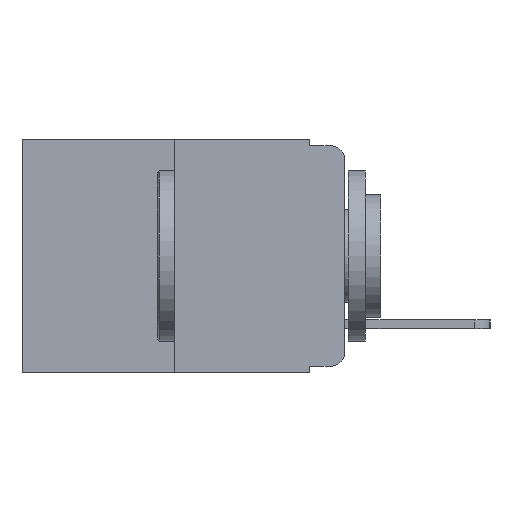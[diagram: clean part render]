
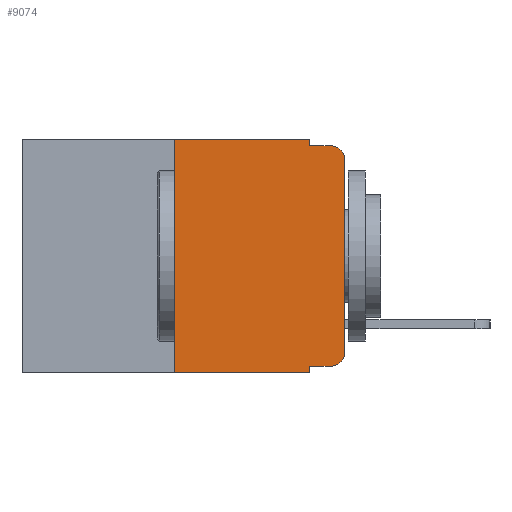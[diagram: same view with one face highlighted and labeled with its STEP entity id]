
A CAD part, left-side view. The second image highlights one B-rep face of the part: STEP entity #9074.
In plain terms, the highlighted planar face has unit normal (-1, 0, 0).
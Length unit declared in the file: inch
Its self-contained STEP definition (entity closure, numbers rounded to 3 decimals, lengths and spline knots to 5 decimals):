
#19 = EDGE_CURVE ( 'NONE', #1099, #6830, #603, .T. ) ;
#603 = LINE ( 'NONE', #7827, #10453 ) ;
#739 = CARTESIAN_POINT ( 'NONE',  ( 0., 0.25, 0. ) ) ;
#1099 = VERTEX_POINT ( 'NONE', #2550 ) ;
#1202 = VECTOR ( 'NONE', #2510, 39.37008 ) ;
#1373 = VERTEX_POINT ( 'NONE', #11990 ) ;
#1437 = CARTESIAN_POINT ( 'NONE',  ( 0., 0.25, 0. ) ) ;
#1465 = DIRECTION ( 'NONE',  ( 0., 0., -1. ) ) ;
#1490 = LINE ( 'NONE', #1537, #1202 ) ;
#1537 = CARTESIAN_POINT ( 'NONE',  ( 0., 0.051, 0. ) ) ;
#1784 = ORIENTED_EDGE ( 'NONE', *, *, #7471, .F. ) ;
#2403 = DIRECTION ( 'NONE',  ( 0., 0., 1. ) ) ;
#2408 = LINE ( 'NONE', #4635, #7190 ) ;
#2483 = VECTOR ( 'NONE', #2403, 39.37008 ) ;
#2510 = DIRECTION ( 'NONE',  ( 0., 0., -1. ) ) ;
#2531 = ORIENTED_EDGE ( 'NONE', *, *, #8270, .F. ) ;
#2550 = CARTESIAN_POINT ( 'NONE',  ( 0., 0.051, -0.333 ) ) ;
#2999 = CARTESIAN_POINT ( 'NONE',  ( 0., 0.051, 0. ) ) ;
#3249 = EDGE_CURVE ( 'NONE', #1373, #6670, #10526, .T. ) ;
#3346 = DIRECTION ( 'NONE',  ( 0., -1., 0. ) ) ;
#3503 = CARTESIAN_POINT ( 'NONE',  ( 0., 0., 0. ) ) ;
#3702 = VERTEX_POINT ( 'NONE', #5982 ) ;
#4160 = VERTEX_POINT ( 'NONE', #11303 ) ;
#4472 = DIRECTION ( 'NONE',  ( 0., 0., 1. ) ) ;
#4635 = CARTESIAN_POINT ( 'NONE',  ( 0., 0.473, -0.343 ) ) ;
#4726 = LINE ( 'NONE', #7606, #11687 ) ;
#4774 = CARTESIAN_POINT ( 'NONE',  ( 0., 0.02, -0.333 ) ) ;
#4879 = DIRECTION ( 'NONE',  ( -1., 0., 0. ) ) ;
#5099 = EDGE_CURVE ( 'NONE', #9216, #3702, #11825, .T. ) ;
#5413 = EDGE_CURVE ( 'NONE', #7577, #1373, #7376, .T. ) ;
#5531 = CARTESIAN_POINT ( 'NONE',  ( 0., 0.02, -0.03 ) ) ;
#5548 = CARTESIAN_POINT ( 'NONE',  ( 0., 0.051, 0. ) ) ;
#5604 = DIRECTION ( 'NONE',  ( -1., 0., 0. ) ) ;
#5615 = AXIS2_PLACEMENT_3D ( 'NONE', #9988, #7196, #1465 ) ;
#5924 = VECTOR ( 'NONE', #9632, 39.37008 ) ;
#5982 = CARTESIAN_POINT ( 'NONE',  ( 0., 0.051, -0.01 ) ) ;
#6276 = DIRECTION ( 'NONE',  ( 0., 0., -1. ) ) ;
#6534 = EDGE_CURVE ( 'NONE', #4160, #9773, #7863, .T. ) ;
#6593 = FACE_OUTER_BOUND ( 'NONE', #11711, .T. ) ;
#6670 = VERTEX_POINT ( 'NONE', #9211 ) ;
#6800 = ORIENTED_EDGE ( 'NONE', *, *, #5413, .T. ) ;
#6830 = VERTEX_POINT ( 'NONE', #4774 ) ;
#7030 = ORIENTED_EDGE ( 'NONE', *, *, #19, .T. ) ;
#7073 = VECTOR ( 'NONE', #4472, 39.37008 ) ;
#7190 = VECTOR ( 'NONE', #11309, 39.37008 ) ;
#7196 = DIRECTION ( 'NONE',  ( 1., 0., 0. ) ) ;
#7376 = LINE ( 'NONE', #3503, #7073 ) ;
#7471 = EDGE_CURVE ( 'NONE', #3702, #6670, #4726, .T. ) ;
#7577 = VERTEX_POINT ( 'NONE', #8160 ) ;
#7606 = CARTESIAN_POINT ( 'NONE',  ( 0., 0.051, -0.01 ) ) ;
#7827 = CARTESIAN_POINT ( 'NONE',  ( 0., 0.051, -0.333 ) ) ;
#7863 = LINE ( 'NONE', #1437, #2483 ) ;
#7909 = ORIENTED_EDGE ( 'NONE', *, *, #5099, .F. ) ;
#8115 = PLANE ( 'NONE',  #5615 ) ;
#8160 = CARTESIAN_POINT ( 'NONE',  ( 0., 0., -0.313 ) ) ;
#8201 = ORIENTED_EDGE ( 'NONE', *, *, #6534, .F. ) ;
#8270 = EDGE_CURVE ( 'NONE', #9773, #9216, #9116, .T. ) ;
#8429 = EDGE_CURVE ( 'NONE', #6830, #7577, #10471, .T. ) ;
#8838 = VECTOR ( 'NONE', #10330, 39.37008 ) ;
#9074 = ADVANCED_FACE ( 'NONE', ( #6593 ), #8115, .F. ) ;
#9116 = LINE ( 'NONE', #9362, #8838 ) ;
#9176 = ORIENTED_EDGE ( 'NONE', *, *, #11615, .F. ) ;
#9211 = CARTESIAN_POINT ( 'NONE',  ( 0., 0.02, -0.01 ) ) ;
#9216 = VERTEX_POINT ( 'NONE', #5548 ) ;
#9362 = CARTESIAN_POINT ( 'NONE',  ( 0., 0.473, 0. ) ) ;
#9632 = DIRECTION ( 'NONE',  ( 0., 0., -1. ) ) ;
#9773 = VERTEX_POINT ( 'NONE', #739 ) ;
#9839 = ORIENTED_EDGE ( 'NONE', *, *, #11104, .T. ) ;
#9932 = CARTESIAN_POINT ( 'NONE',  ( 0., 0.051, -0.343 ) ) ;
#9988 = CARTESIAN_POINT ( 'NONE',  ( 0., 0.473, 0. ) ) ;
#10299 = ORIENTED_EDGE ( 'NONE', *, *, #8429, .T. ) ;
#10330 = DIRECTION ( 'NONE',  ( 0., -1., 0. ) ) ;
#10453 = VECTOR ( 'NONE', #3346, 39.37008 ) ;
#10458 = DIRECTION ( 'NONE',  ( 0., -1., 0. ) ) ;
#10471 = CIRCLE ( 'NONE', #11402, 0.02 ) ;
#10497 = AXIS2_PLACEMENT_3D ( 'NONE', #5531, #5604, #6276 ) ;
#10519 = ORIENTED_EDGE ( 'NONE', *, *, #3249, .T. ) ;
#10526 = CIRCLE ( 'NONE', #10497, 0.02 ) ;
#10543 = CARTESIAN_POINT ( 'NONE',  ( 0., 0.02, -0.313 ) ) ;
#11104 = EDGE_CURVE ( 'NONE', #4160, #11530, #2408, .T. ) ;
#11303 = CARTESIAN_POINT ( 'NONE',  ( 0., 0.25, -0.343 ) ) ;
#11309 = DIRECTION ( 'NONE',  ( 0., -1., 0. ) ) ;
#11402 = AXIS2_PLACEMENT_3D ( 'NONE', #10543, #4879, #11504 ) ;
#11504 = DIRECTION ( 'NONE',  ( 0., 0., -1. ) ) ;
#11530 = VERTEX_POINT ( 'NONE', #9932 ) ;
#11615 = EDGE_CURVE ( 'NONE', #1099, #11530, #1490, .T. ) ;
#11687 = VECTOR ( 'NONE', #10458, 39.37008 ) ;
#11711 = EDGE_LOOP ( 'NONE', ( #6800, #10519, #1784, #7909, #2531, #8201, #9839, #9176, #7030, #10299 ) ) ;
#11825 = LINE ( 'NONE', #2999, #5924 ) ;
#11990 = CARTESIAN_POINT ( 'NONE',  ( 0., 0., -0.03 ) ) ;
